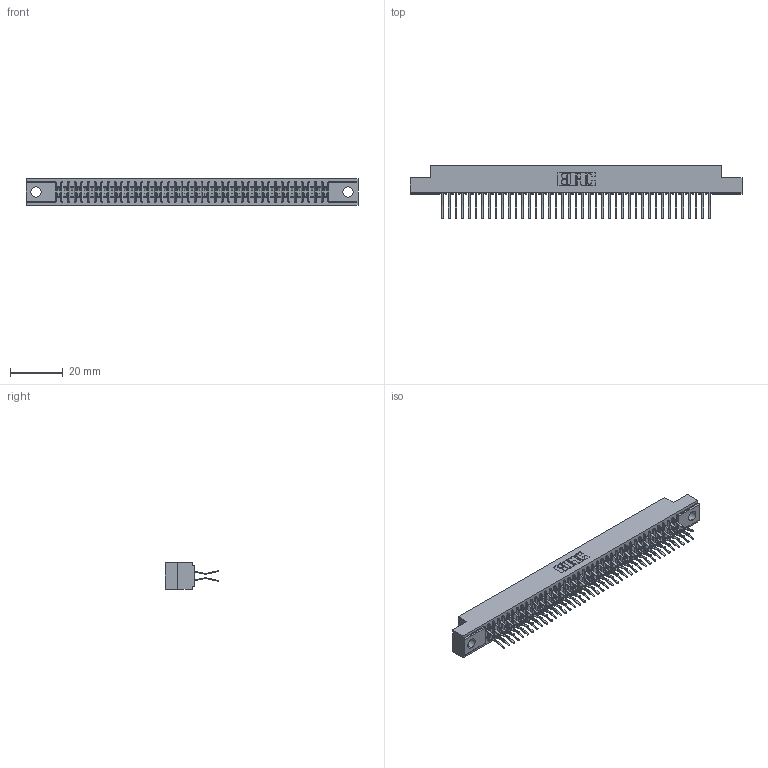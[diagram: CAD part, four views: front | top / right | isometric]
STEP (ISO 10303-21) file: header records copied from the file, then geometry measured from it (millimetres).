
FILE_DESCRIPTION (( 'STEP AP203' ), '1' );
FILE_NAME ('391-082-560-204.STEP', '2018-08-09T16:11:06', ( '' ), ( '' ), 'SwSTEP 2.0', 'SolidWorks 2016', '' );
FILE_SCHEMA (( 'CONFIG_CONTROL_DESIGN' ));
Length unit declared in the file: inch
Products named in the file (3): 391-082-560-204; 341 Part_.156 (3.96) Dia Mounting Holes; 341-292-001_341-292-160
Assembly tree (83 placements, depth 2):
  391-082-560-204
    341 Part_.156 (3.96) Dia Mounting Holes
    341-292-001_341-292-160  x82
Bounding box: 126.36 x 20.37 x 10.16 mm (x, y, z)
Volume: 9306 mm3; surface area: 16981.1 mm2
Topology: 83 solids, 83 shells, 5870 faces, 17039 edges, 11054 vertices
Faces by surface type: plane 3362, cylinder 2344, sphere 84, torus 80
Entity records: 50310 total; most frequent: CARTESIAN_POINT 8369, ORIENTED_EDGE 8314, DIRECTION 8119, EDGE_CURVE 4157, LINE 3359, VECTOR 3359, VERTEX_POINT 2630, AXIS2_PLACEMENT_3D 2380
